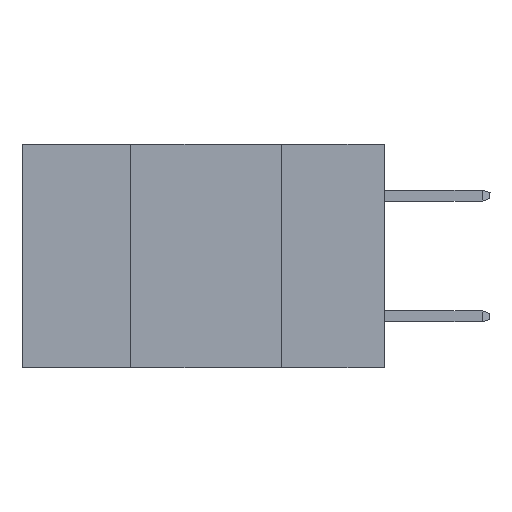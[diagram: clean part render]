
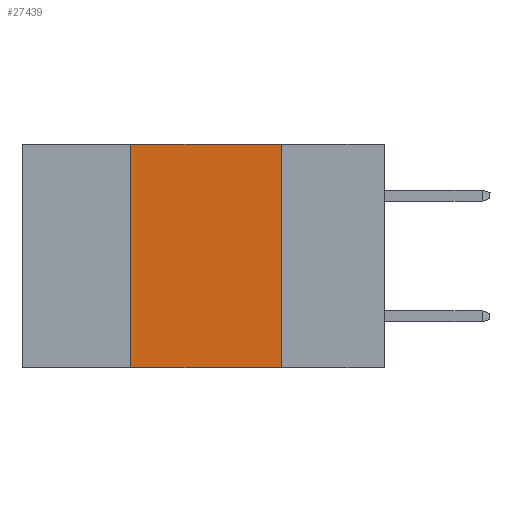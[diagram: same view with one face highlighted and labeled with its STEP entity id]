
A CAD part, left-side view. The second image highlights one B-rep face of the part: STEP entity #27439.
In plain terms, the highlighted planar face has unit normal (-1, 0, 0).
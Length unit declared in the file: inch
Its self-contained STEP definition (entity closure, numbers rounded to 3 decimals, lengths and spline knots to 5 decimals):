
#763 = ORIENTED_EDGE ( 'NONE', *, *, #29013, .F. ) ;
#2584 = EDGE_CURVE ( 'NONE', #25412, #3274, #23824, .T. ) ;
#2736 = DIRECTION ( 'NONE',  ( 0., 0., -1. ) ) ;
#3193 = CARTESIAN_POINT ( 'NONE',  ( 0., 0.17, 0. ) ) ;
#3274 = VERTEX_POINT ( 'NONE', #23097 ) ;
#3277 = DIRECTION ( 'NONE',  ( 0., -1., 0. ) ) ;
#5238 = VECTOR ( 'NONE', #3277, 39.37008 ) ;
#7013 = VERTEX_POINT ( 'NONE', #3193 ) ;
#7707 = EDGE_CURVE ( 'NONE', #25412, #26861, #20732, .T. ) ;
#7860 = VECTOR ( 'NONE', #21753, 39.37008 ) ;
#10503 = ORIENTED_EDGE ( 'NONE', *, *, #30468, .F. ) ;
#11045 = AXIS2_PLACEMENT_3D ( 'NONE', #24133, #31069, #24036 ) ;
#12250 = DIRECTION ( 'NONE',  ( 0., -1., 0. ) ) ;
#12786 = CARTESIAN_POINT ( 'NONE',  ( 0., 0.17, 0. ) ) ;
#14327 = LINE ( 'NONE', #22020, #19246 ) ;
#16725 = LINE ( 'NONE', #12786, #18594 ) ;
#17631 = FACE_OUTER_BOUND ( 'NONE', #28970, .T. ) ;
#17641 = CARTESIAN_POINT ( 'NONE',  ( 0., 0.42, 0. ) ) ;
#18594 = VECTOR ( 'NONE', #2736, 39.37008 ) ;
#19246 = VECTOR ( 'NONE', #12250, 39.37008 ) ;
#19499 = CARTESIAN_POINT ( 'NONE',  ( 0., 0.42, 0. ) ) ;
#20732 = LINE ( 'NONE', #19499, #7860 ) ;
#21753 = DIRECTION ( 'NONE',  ( 0., 0., 1. ) ) ;
#22020 = CARTESIAN_POINT ( 'NONE',  ( 0., 0.6, 0. ) ) ;
#23003 = ORIENTED_EDGE ( 'NONE', *, *, #7707, .F. ) ;
#23069 = ORIENTED_EDGE ( 'NONE', *, *, #2584, .T. ) ;
#23097 = CARTESIAN_POINT ( 'NONE',  ( 0., 0.17, -0.37 ) ) ;
#23824 = LINE ( 'NONE', #29976, #5238 ) ;
#24036 = DIRECTION ( 'NONE',  ( 0., 0., -1. ) ) ;
#24133 = CARTESIAN_POINT ( 'NONE',  ( 0., 0.6, 0. ) ) ;
#25412 = VERTEX_POINT ( 'NONE', #30868 ) ;
#26861 = VERTEX_POINT ( 'NONE', #17641 ) ;
#27439 = ADVANCED_FACE ( 'NONE', ( #17631 ), #28930, .F. ) ;
#28930 = PLANE ( 'NONE',  #11045 ) ;
#28970 = EDGE_LOOP ( 'NONE', ( #763, #10503, #23003, #23069 ) ) ;
#29013 = EDGE_CURVE ( 'NONE', #7013, #3274, #16725, .T. ) ;
#29976 = CARTESIAN_POINT ( 'NONE',  ( 0., 0.6, -0.37 ) ) ;
#30468 = EDGE_CURVE ( 'NONE', #26861, #7013, #14327, .T. ) ;
#30868 = CARTESIAN_POINT ( 'NONE',  ( 0., 0.42, -0.37 ) ) ;
#31069 = DIRECTION ( 'NONE',  ( 1., 0., 0. ) ) ;
